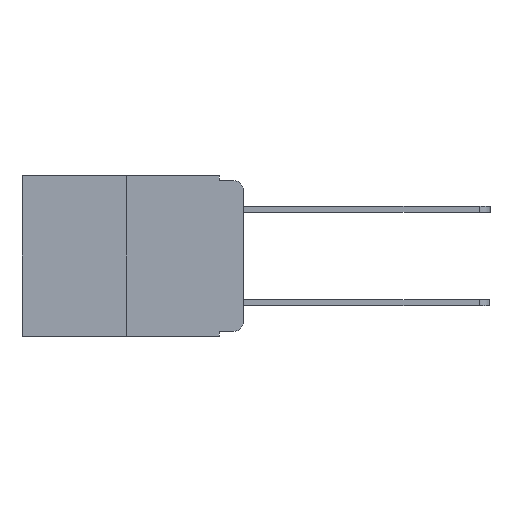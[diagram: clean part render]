
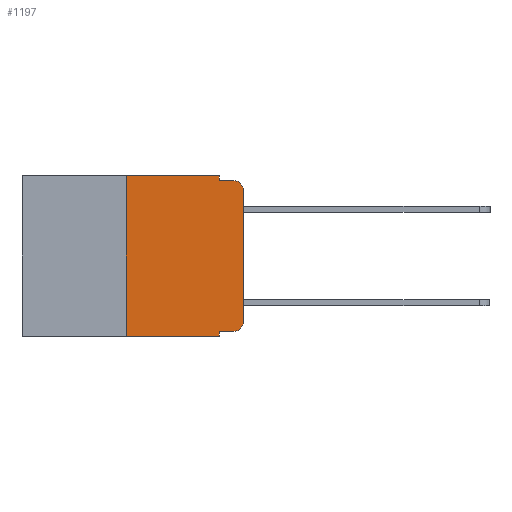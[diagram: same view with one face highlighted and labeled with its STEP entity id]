
A CAD part, left-side view. The second image highlights one B-rep face of the part: STEP entity #1197.
In plain terms, the highlighted planar face has unit normal (-1, 0, 0).
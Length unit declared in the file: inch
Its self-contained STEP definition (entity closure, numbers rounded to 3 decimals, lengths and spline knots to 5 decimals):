
#291 = CARTESIAN_POINT ( 'NONE',  ( 0., 0., -0.313 ) ) ;
#579 = VECTOR ( 'NONE', #7603, 39.37008 ) ;
#745 = ORIENTED_EDGE ( 'NONE', *, *, #1786, .F. ) ;
#1001 = VECTOR ( 'NONE', #8900, 39.37008 ) ;
#1012 = VERTEX_POINT ( 'NONE', #291 ) ;
#1158 = EDGE_LOOP ( 'NONE', ( #19133, #4416, #7494, #745, #8859, #13249, #6273, #4684, #16414, #9581 ) ) ;
#1197 = ADVANCED_FACE ( 'NONE', ( #2033 ), #11710, .F. ) ;
#1201 = DIRECTION ( 'NONE',  ( 0., -1., 0. ) ) ;
#1674 = CIRCLE ( 'NONE', #15178, 0.02 ) ;
#1786 = EDGE_CURVE ( 'NONE', #1994, #4398, #16870, .T. ) ;
#1994 = VERTEX_POINT ( 'NONE', #6429 ) ;
#2033 = FACE_OUTER_BOUND ( 'NONE', #1158, .T. ) ;
#2221 = DIRECTION ( 'NONE',  ( 0., 0., -1. ) ) ;
#2816 = EDGE_CURVE ( 'NONE', #4398, #7434, #3157, .T. ) ;
#3157 = LINE ( 'NONE', #9659, #3670 ) ;
#3296 = VERTEX_POINT ( 'NONE', #8160 ) ;
#3555 = CARTESIAN_POINT ( 'NONE',  ( 0., 0., -0.03 ) ) ;
#3670 = VECTOR ( 'NONE', #15455, 39.37008 ) ;
#3885 = EDGE_CURVE ( 'NONE', #18592, #7434, #1674, .T. ) ;
#4398 = VERTEX_POINT ( 'NONE', #5033 ) ;
#4416 = ORIENTED_EDGE ( 'NONE', *, *, #3885, .T. ) ;
#4684 = ORIENTED_EDGE ( 'NONE', *, *, #17100, .F. ) ;
#4752 = LINE ( 'NONE', #14888, #579 ) ;
#4900 = EDGE_CURVE ( 'NONE', #1012, #18592, #18132, .T. ) ;
#5033 = CARTESIAN_POINT ( 'NONE',  ( 0., 0.051, -0.01 ) ) ;
#5476 = LINE ( 'NONE', #8791, #16731 ) ;
#5911 = LINE ( 'NONE', #6841, #8928 ) ;
#6273 = ORIENTED_EDGE ( 'NONE', *, *, #11497, .T. ) ;
#6429 = CARTESIAN_POINT ( 'NONE',  ( 0., 0.051, 0. ) ) ;
#6841 = CARTESIAN_POINT ( 'NONE',  ( 0., 0.051, 0. ) ) ;
#7224 = AXIS2_PLACEMENT_3D ( 'NONE', #17067, #8321, #18543 ) ;
#7434 = VERTEX_POINT ( 'NONE', #10939 ) ;
#7494 = ORIENTED_EDGE ( 'NONE', *, *, #2816, .F. ) ;
#7603 = DIRECTION ( 'NONE',  ( 0., -1., 0. ) ) ;
#8011 = CARTESIAN_POINT ( 'NONE',  ( 0., 0., 0. ) ) ;
#8160 = CARTESIAN_POINT ( 'NONE',  ( 0., 0.25, -0.343 ) ) ;
#8207 = DIRECTION ( 'NONE',  ( -1., 0., 0. ) ) ;
#8222 = VECTOR ( 'NONE', #14860, 39.37008 ) ;
#8321 = DIRECTION ( 'NONE',  ( -1., 0., 0. ) ) ;
#8791 = CARTESIAN_POINT ( 'NONE',  ( 0., 0.051, -0.333 ) ) ;
#8859 = ORIENTED_EDGE ( 'NONE', *, *, #10774, .F. ) ;
#8900 = DIRECTION ( 'NONE',  ( 0., 0., -1. ) ) ;
#8928 = VECTOR ( 'NONE', #2221, 39.37008 ) ;
#9103 = CARTESIAN_POINT ( 'NONE',  ( 0., 0.25, 0. ) ) ;
#9275 = AXIS2_PLACEMENT_3D ( 'NONE', #17739, #12265, #10966 ) ;
#9581 = ORIENTED_EDGE ( 'NONE', *, *, #15145, .T. ) ;
#9659 = CARTESIAN_POINT ( 'NONE',  ( 0., 0.051, -0.01 ) ) ;
#10272 = DIRECTION ( 'NONE',  ( 0., -1., 0. ) ) ;
#10383 = VECTOR ( 'NONE', #16736, 39.37008 ) ;
#10774 = EDGE_CURVE ( 'NONE', #11187, #1994, #17201, .T. ) ;
#10792 = VERTEX_POINT ( 'NONE', #17592 ) ;
#10939 = CARTESIAN_POINT ( 'NONE',  ( 0., 0.02, -0.01 ) ) ;
#10966 = DIRECTION ( 'NONE',  ( 0., 0., -1. ) ) ;
#11187 = VERTEX_POINT ( 'NONE', #11222 ) ;
#11222 = CARTESIAN_POINT ( 'NONE',  ( 0., 0.25, 0. ) ) ;
#11497 = EDGE_CURVE ( 'NONE', #3296, #10792, #4752, .T. ) ;
#11710 = PLANE ( 'NONE',  #9275 ) ;
#12265 = DIRECTION ( 'NONE',  ( 1., 0., 0. ) ) ;
#12595 = LINE ( 'NONE', #9103, #8222 ) ;
#13249 = ORIENTED_EDGE ( 'NONE', *, *, #19051, .F. ) ;
#13355 = VECTOR ( 'NONE', #10272, 39.37008 ) ;
#13693 = VERTEX_POINT ( 'NONE', #18400 ) ;
#14287 = CIRCLE ( 'NONE', #7224, 0.02 ) ;
#14608 = CARTESIAN_POINT ( 'NONE',  ( 0., 0.473, 0. ) ) ;
#14788 = CARTESIAN_POINT ( 'NONE',  ( 0., 0.051, 0. ) ) ;
#14860 = DIRECTION ( 'NONE',  ( 0., 0., 1. ) ) ;
#14888 = CARTESIAN_POINT ( 'NONE',  ( 0., 0.473, -0.343 ) ) ;
#15145 = EDGE_CURVE ( 'NONE', #16563, #1012, #14287, .T. ) ;
#15178 = AXIS2_PLACEMENT_3D ( 'NONE', #16955, #8207, #18419 ) ;
#15455 = DIRECTION ( 'NONE',  ( 0., -1., 0. ) ) ;
#16109 = EDGE_CURVE ( 'NONE', #13693, #16563, #5476, .T. ) ;
#16414 = ORIENTED_EDGE ( 'NONE', *, *, #16109, .T. ) ;
#16563 = VERTEX_POINT ( 'NONE', #17149 ) ;
#16731 = VECTOR ( 'NONE', #1201, 39.37008 ) ;
#16736 = DIRECTION ( 'NONE',  ( 0., 0., 1. ) ) ;
#16870 = LINE ( 'NONE', #14788, #1001 ) ;
#16955 = CARTESIAN_POINT ( 'NONE',  ( 0., 0.02, -0.03 ) ) ;
#17067 = CARTESIAN_POINT ( 'NONE',  ( 0., 0.02, -0.313 ) ) ;
#17100 = EDGE_CURVE ( 'NONE', #13693, #10792, #5911, .T. ) ;
#17149 = CARTESIAN_POINT ( 'NONE',  ( 0., 0.02, -0.333 ) ) ;
#17201 = LINE ( 'NONE', #14608, #13355 ) ;
#17592 = CARTESIAN_POINT ( 'NONE',  ( 0., 0.051, -0.343 ) ) ;
#17739 = CARTESIAN_POINT ( 'NONE',  ( 0., 0.473, 0. ) ) ;
#18132 = LINE ( 'NONE', #8011, #10383 ) ;
#18400 = CARTESIAN_POINT ( 'NONE',  ( 0., 0.051, -0.333 ) ) ;
#18419 = DIRECTION ( 'NONE',  ( 0., 0., -1. ) ) ;
#18543 = DIRECTION ( 'NONE',  ( 0., 0., -1. ) ) ;
#18592 = VERTEX_POINT ( 'NONE', #3555 ) ;
#19051 = EDGE_CURVE ( 'NONE', #3296, #11187, #12595, .T. ) ;
#19133 = ORIENTED_EDGE ( 'NONE', *, *, #4900, .T. ) ;
